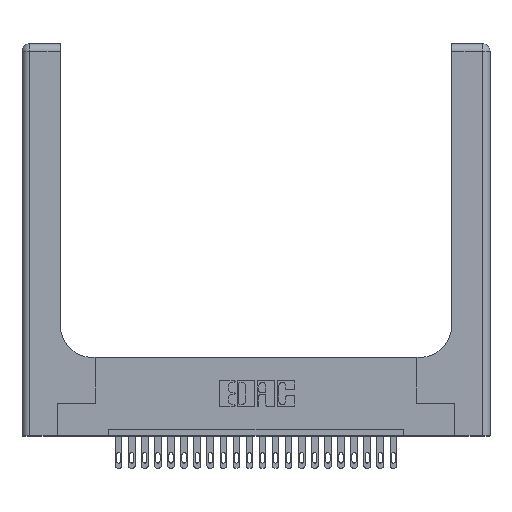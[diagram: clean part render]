
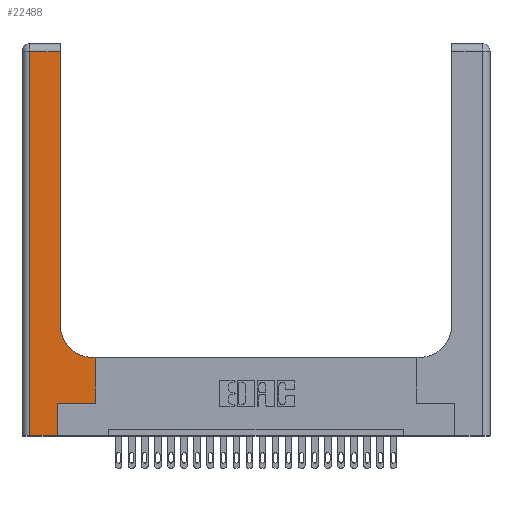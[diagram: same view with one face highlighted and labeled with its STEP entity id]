
A CAD part, top view. The second image highlights one B-rep face of the part: STEP entity #22488.
In plain terms, the highlighted planar face has unit normal (0, 0, 1).
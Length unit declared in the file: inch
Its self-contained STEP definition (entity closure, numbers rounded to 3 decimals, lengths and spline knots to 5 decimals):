
#436 = DIRECTION ( 'NONE',  ( 0., 1., 0. ) ) ;
#1057 = EDGE_CURVE ( 'NONE', #9896, #13633, #17270, .T. ) ;
#1092 = CARTESIAN_POINT ( 'NONE',  ( 0.269, 0.25, 0.37 ) ) ;
#1259 = VERTEX_POINT ( 'NONE', #24173 ) ;
#1738 = CARTESIAN_POINT ( 'NONE',  ( 0.06, 2.94, 0.37 ) ) ;
#1991 = EDGE_CURVE ( 'NONE', #3913, #7339, #16404, .T. ) ;
#2083 = CIRCLE ( 'NONE', #7018, 0.25 ) ;
#2299 = EDGE_CURVE ( 'NONE', #19534, #9896, #6079, .T. ) ;
#2775 = DIRECTION ( 'NONE',  ( 0., 1., 0. ) ) ;
#3068 = ORIENTED_EDGE ( 'NONE', *, *, #4740, .T. ) ;
#3643 = ORIENTED_EDGE ( 'NONE', *, *, #17198, .T. ) ;
#3657 = DIRECTION ( 'NONE',  ( 0., 0., -1. ) ) ;
#3708 = CARTESIAN_POINT ( 'NONE',  ( 0.269, 0.25, 0.37 ) ) ;
#3878 = VERTEX_POINT ( 'NONE', #18585 ) ;
#3913 = VERTEX_POINT ( 'NONE', #7174 ) ;
#3978 = DIRECTION ( 'NONE',  ( -1., 0., 0. ) ) ;
#4304 = LINE ( 'NONE', #9691, #19570 ) ;
#4418 = LINE ( 'NONE', #13238, #13256 ) ;
#4633 = ORIENTED_EDGE ( 'NONE', *, *, #14869, .T. ) ;
#4740 = EDGE_CURVE ( 'NONE', #18770, #3878, #2083, .T. ) ;
#4933 = DIRECTION ( 'NONE',  ( 0., -1., 0. ) ) ;
#5515 = ORIENTED_EDGE ( 'NONE', *, *, #18136, .T. ) ;
#5996 = CARTESIAN_POINT ( 'NONE',  ( 0.5415, 0.6, 0.37 ) ) ;
#6032 = DIRECTION ( 'NONE',  ( 0., 0., -1. ) ) ;
#6079 = LINE ( 'NONE', #3708, #22254 ) ;
#6467 = VERTEX_POINT ( 'NONE', #19409 ) ;
#6938 = CARTESIAN_POINT ( 'NONE',  ( 0., 2.94, 0.37 ) ) ;
#7018 = AXIS2_PLACEMENT_3D ( 'NONE', #18089, #6032, #21063 ) ;
#7174 = CARTESIAN_POINT ( 'NONE',  ( 0.2915, 2.94, 0.37 ) ) ;
#7339 = VERTEX_POINT ( 'NONE', #1738 ) ;
#7832 = CARTESIAN_POINT ( 'NONE',  ( 0.5585, 0.25, 0.37 ) ) ;
#7979 = DIRECTION ( 'NONE',  ( 0., 1., 0. ) ) ;
#9042 = VECTOR ( 'NONE', #15870, 39.37008 ) ;
#9691 = CARTESIAN_POINT ( 'NONE',  ( 0.269, 0., 0.37 ) ) ;
#9896 = VERTEX_POINT ( 'NONE', #7832 ) ;
#11228 = CARTESIAN_POINT ( 'NONE',  ( 0., 3., 0.37 ) ) ;
#11385 = VECTOR ( 'NONE', #7979, 39.37008 ) ;
#12033 = FACE_OUTER_BOUND ( 'NONE', #21828, .T. ) ;
#12607 = VECTOR ( 'NONE', #2775, 39.37008 ) ;
#12706 = ORIENTED_EDGE ( 'NONE', *, *, #18835, .T. ) ;
#13238 = CARTESIAN_POINT ( 'NONE',  ( 0.06, 3., 0.37 ) ) ;
#13256 = VECTOR ( 'NONE', #4933, 39.37008 ) ;
#13558 = CARTESIAN_POINT ( 'NONE',  ( 0.5585, 0.25, 0.37 ) ) ;
#13595 = LINE ( 'NONE', #20246, #16533 ) ;
#13633 = VERTEX_POINT ( 'NONE', #19729 ) ;
#14554 = VECTOR ( 'NONE', #21156, 39.37008 ) ;
#14869 = EDGE_CURVE ( 'NONE', #6467, #19534, #4304, .T. ) ;
#15475 = ORIENTED_EDGE ( 'NONE', *, *, #23176, .T. ) ;
#15512 = CARTESIAN_POINT ( 'NONE',  ( 0., 0., 0.37 ) ) ;
#15870 = DIRECTION ( 'NONE',  ( -1., 0., 0. ) ) ;
#16404 = LINE ( 'NONE', #6938, #9042 ) ;
#16533 = VECTOR ( 'NONE', #20491, 39.37008 ) ;
#16689 = LINE ( 'NONE', #21449, #12607 ) ;
#16742 = ORIENTED_EDGE ( 'NONE', *, *, #2299, .T. ) ;
#17198 = EDGE_CURVE ( 'NONE', #1259, #6467, #19504, .T. ) ;
#17270 = LINE ( 'NONE', #13558, #11385 ) ;
#17506 = ORIENTED_EDGE ( 'NONE', *, *, #1991, .T. ) ;
#18089 = CARTESIAN_POINT ( 'NONE',  ( 0.5415, 0.85, 0.37 ) ) ;
#18136 = EDGE_CURVE ( 'NONE', #13633, #18770, #13595, .T. ) ;
#18585 = CARTESIAN_POINT ( 'NONE',  ( 0.2915, 0.85, 0.37 ) ) ;
#18770 = VERTEX_POINT ( 'NONE', #5996 ) ;
#18835 = EDGE_CURVE ( 'NONE', #7339, #1259, #4418, .T. ) ;
#19409 = CARTESIAN_POINT ( 'NONE',  ( 0.269, 0., 0.37 ) ) ;
#19504 = LINE ( 'NONE', #15512, #14554 ) ;
#19534 = VERTEX_POINT ( 'NONE', #1092 ) ;
#19570 = VECTOR ( 'NONE', #436, 39.37008 ) ;
#19729 = CARTESIAN_POINT ( 'NONE',  ( 0.5585, 0.6, 0.37 ) ) ;
#20246 = CARTESIAN_POINT ( 'NONE',  ( 0.2915, 0.6, 0.37 ) ) ;
#20491 = DIRECTION ( 'NONE',  ( -1., 0., 0. ) ) ;
#20645 = DIRECTION ( 'NONE',  ( 1., 0., 0. ) ) ;
#21063 = DIRECTION ( 'NONE',  ( 1., 0., 0. ) ) ;
#21156 = DIRECTION ( 'NONE',  ( 1., 0., 0. ) ) ;
#21449 = CARTESIAN_POINT ( 'NONE',  ( 0.2915, 3., 0.37 ) ) ;
#21828 = EDGE_LOOP ( 'NONE', ( #15475, #17506, #12706, #3643, #4633, #16742, #22757, #5515, #3068 ) ) ;
#22254 = VECTOR ( 'NONE', #20645, 39.37008 ) ;
#22488 = ADVANCED_FACE ( 'NONE', ( #12033 ), #22715, .F. ) ;
#22715 = PLANE ( 'NONE',  #24066 ) ;
#22757 = ORIENTED_EDGE ( 'NONE', *, *, #1057, .T. ) ;
#23176 = EDGE_CURVE ( 'NONE', #3878, #3913, #16689, .T. ) ;
#24066 = AXIS2_PLACEMENT_3D ( 'NONE', #11228, #3657, #3978 ) ;
#24173 = CARTESIAN_POINT ( 'NONE',  ( 0.06, 0., 0.37 ) ) ;
